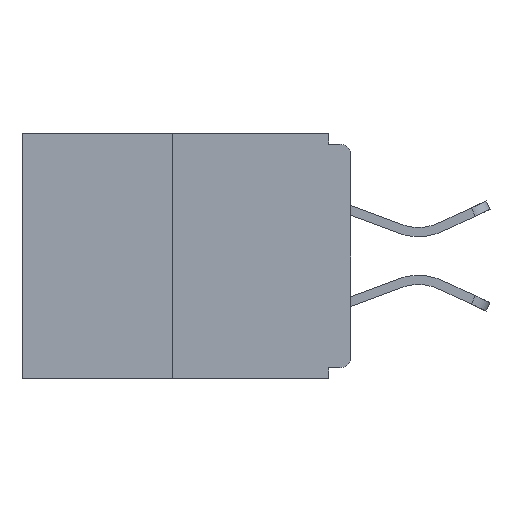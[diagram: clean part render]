
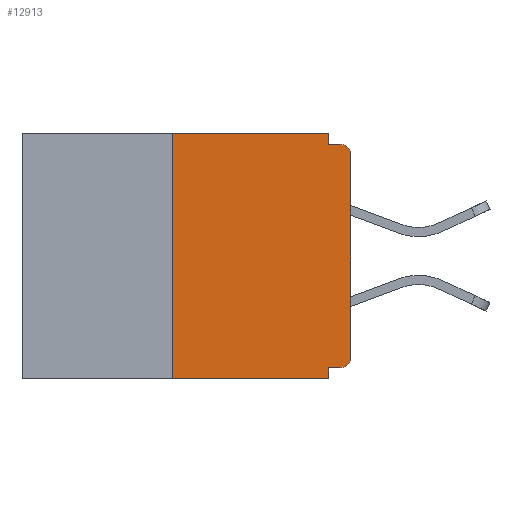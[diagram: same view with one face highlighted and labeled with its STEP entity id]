
A CAD part, left-side view. The second image highlights one B-rep face of the part: STEP entity #12913.
In plain terms, the highlighted planar face has unit normal (-1, 0, 0).
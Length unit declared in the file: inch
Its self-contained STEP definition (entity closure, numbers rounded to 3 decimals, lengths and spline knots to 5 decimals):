
#12 = FACE_OUTER_BOUND ( 'NONE', #16974, .T. ) ;
#173 = AXIS2_PLACEMENT_3D ( 'NONE', #5861, #2573, #17564 ) ;
#199 = EDGE_CURVE ( 'NONE', #420, #7550, #18023, .T. ) ;
#322 = CARTESIAN_POINT ( 'NONE',  ( 0., 0.031, -0.343 ) ) ;
#420 = VERTEX_POINT ( 'NONE', #993 ) ;
#993 = CARTESIAN_POINT ( 'NONE',  ( 0., 0.015, -0.328 ) ) ;
#1080 = ORIENTED_EDGE ( 'NONE', *, *, #20466, .F. ) ;
#1146 = DIRECTION ( 'NONE',  ( 0., 0., 1. ) ) ;
#1166 = AXIS2_PLACEMENT_3D ( 'NONE', #9513, #14230, #17580 ) ;
#1362 = ORIENTED_EDGE ( 'NONE', *, *, #5950, .F. ) ;
#1486 = ORIENTED_EDGE ( 'NONE', *, *, #1504, .T. ) ;
#1504 = EDGE_CURVE ( 'NONE', #16316, #15945, #9308, .T. ) ;
#1611 = LINE ( 'NONE', #3423, #20469 ) ;
#2573 = DIRECTION ( 'NONE',  ( 1., 0., 0. ) ) ;
#2588 = LINE ( 'NONE', #8252, #7554 ) ;
#3042 = VERTEX_POINT ( 'NONE', #17870 ) ;
#3053 = DIRECTION ( 'NONE',  ( 0., -1., 0. ) ) ;
#3219 = ORIENTED_EDGE ( 'NONE', *, *, #11338, .T. ) ;
#3356 = DIRECTION ( 'NONE',  ( 0., -1., 0. ) ) ;
#3362 = DIRECTION ( 'NONE',  ( 0., -1., 0. ) ) ;
#3423 = CARTESIAN_POINT ( 'NONE',  ( 0., 0.46, -0.343 ) ) ;
#3462 = CARTESIAN_POINT ( 'NONE',  ( 0., 0.031, -0.015 ) ) ;
#3541 = VECTOR ( 'NONE', #3362, 39.37008 ) ;
#3561 = VECTOR ( 'NONE', #3053, 39.37008 ) ;
#3677 = CARTESIAN_POINT ( 'NONE',  ( 0., 0.25, 0. ) ) ;
#3780 = VECTOR ( 'NONE', #15400, 39.37008 ) ;
#4090 = LINE ( 'NONE', #9828, #3561 ) ;
#4289 = CARTESIAN_POINT ( 'NONE',  ( 0., 0.031, 0. ) ) ;
#4687 = VERTEX_POINT ( 'NONE', #5733 ) ;
#5733 = CARTESIAN_POINT ( 'NONE',  ( 0., 0.031, -0.343 ) ) ;
#5827 = ORIENTED_EDGE ( 'NONE', *, *, #20928, .F. ) ;
#5861 = CARTESIAN_POINT ( 'NONE',  ( 0., 0.46, 0. ) ) ;
#5950 = EDGE_CURVE ( 'NONE', #17521, #15945, #7951, .T. ) ;
#6357 = LINE ( 'NONE', #15813, #10531 ) ;
#6483 = AXIS2_PLACEMENT_3D ( 'NONE', #17010, #10203, #18713 ) ;
#6975 = CARTESIAN_POINT ( 'NONE',  ( 0., 0., -0.03 ) ) ;
#7078 = VERTEX_POINT ( 'NONE', #3677 ) ;
#7172 = EDGE_CURVE ( 'NONE', #8802, #17521, #6357, .T. ) ;
#7550 = VERTEX_POINT ( 'NONE', #17320 ) ;
#7554 = VECTOR ( 'NONE', #19961, 39.37008 ) ;
#7951 = LINE ( 'NONE', #13214, #3541 ) ;
#8252 = CARTESIAN_POINT ( 'NONE',  ( 0., 0., 0. ) ) ;
#8792 = LINE ( 'NONE', #13596, #10082 ) ;
#8802 = VERTEX_POINT ( 'NONE', #4289 ) ;
#9047 = CARTESIAN_POINT ( 'NONE',  ( 0., 0.015, -0.015 ) ) ;
#9308 = CIRCLE ( 'NONE', #1166, 0.015 ) ;
#9513 = CARTESIAN_POINT ( 'NONE',  ( 0., 0.015, -0.03 ) ) ;
#9828 = CARTESIAN_POINT ( 'NONE',  ( 0., 0.46, 0. ) ) ;
#10082 = VECTOR ( 'NONE', #13674, 39.37008 ) ;
#10203 = DIRECTION ( 'NONE',  ( -1., 0., 0. ) ) ;
#10531 = VECTOR ( 'NONE', #18891, 39.37008 ) ;
#10820 = LINE ( 'NONE', #322, #3780 ) ;
#11338 = EDGE_CURVE ( 'NONE', #3042, #4687, #1611, .T. ) ;
#12580 = PLANE ( 'NONE',  #173 ) ;
#12658 = ORIENTED_EDGE ( 'NONE', *, *, #199, .T. ) ;
#12913 = ADVANCED_FACE ( 'NONE', ( #12 ), #12580, .F. ) ;
#12961 = ORIENTED_EDGE ( 'NONE', *, *, #18783, .T. ) ;
#13214 = CARTESIAN_POINT ( 'NONE',  ( 0., 0., -0.015 ) ) ;
#13596 = CARTESIAN_POINT ( 'NONE',  ( 0., 0., -0.328 ) ) ;
#13674 = DIRECTION ( 'NONE',  ( 0., 1., 0. ) ) ;
#14230 = DIRECTION ( 'NONE',  ( -1., 0., 0. ) ) ;
#14807 = CARTESIAN_POINT ( 'NONE',  ( 0., 0.031, -0.328 ) ) ;
#15400 = DIRECTION ( 'NONE',  ( 0., 0., -1. ) ) ;
#15813 = CARTESIAN_POINT ( 'NONE',  ( 0., 0.031, 0. ) ) ;
#15945 = VERTEX_POINT ( 'NONE', #9047 ) ;
#16316 = VERTEX_POINT ( 'NONE', #6975 ) ;
#16473 = EDGE_CURVE ( 'NONE', #17451, #4687, #10820, .T. ) ;
#16480 = VECTOR ( 'NONE', #1146, 39.37008 ) ;
#16974 = EDGE_LOOP ( 'NONE', ( #1080, #19888, #3219, #19510, #5827, #12658, #12961, #1486, #1362, #18934 ) ) ;
#17010 = CARTESIAN_POINT ( 'NONE',  ( 0., 0.015, -0.313 ) ) ;
#17320 = CARTESIAN_POINT ( 'NONE',  ( 0., 0., -0.313 ) ) ;
#17451 = VERTEX_POINT ( 'NONE', #14807 ) ;
#17521 = VERTEX_POINT ( 'NONE', #3462 ) ;
#17564 = DIRECTION ( 'NONE',  ( 0., 0., -1. ) ) ;
#17580 = DIRECTION ( 'NONE',  ( 0., 0., -1. ) ) ;
#17870 = CARTESIAN_POINT ( 'NONE',  ( 0., 0.25, -0.343 ) ) ;
#18023 = CIRCLE ( 'NONE', #6483, 0.015 ) ;
#18289 = EDGE_CURVE ( 'NONE', #3042, #7078, #20934, .T. ) ;
#18713 = DIRECTION ( 'NONE',  ( 0., 0., -1. ) ) ;
#18783 = EDGE_CURVE ( 'NONE', #7550, #16316, #2588, .T. ) ;
#18891 = DIRECTION ( 'NONE',  ( 0., 0., -1. ) ) ;
#18934 = ORIENTED_EDGE ( 'NONE', *, *, #7172, .F. ) ;
#19431 = CARTESIAN_POINT ( 'NONE',  ( 0., 0.25, 0. ) ) ;
#19510 = ORIENTED_EDGE ( 'NONE', *, *, #16473, .F. ) ;
#19888 = ORIENTED_EDGE ( 'NONE', *, *, #18289, .F. ) ;
#19961 = DIRECTION ( 'NONE',  ( 0., 0., 1. ) ) ;
#20466 = EDGE_CURVE ( 'NONE', #7078, #8802, #4090, .T. ) ;
#20469 = VECTOR ( 'NONE', #3356, 39.37008 ) ;
#20928 = EDGE_CURVE ( 'NONE', #420, #17451, #8792, .T. ) ;
#20934 = LINE ( 'NONE', #19431, #16480 ) ;
